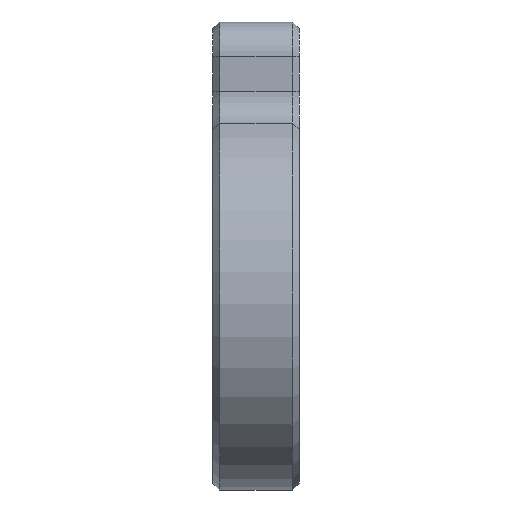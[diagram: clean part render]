
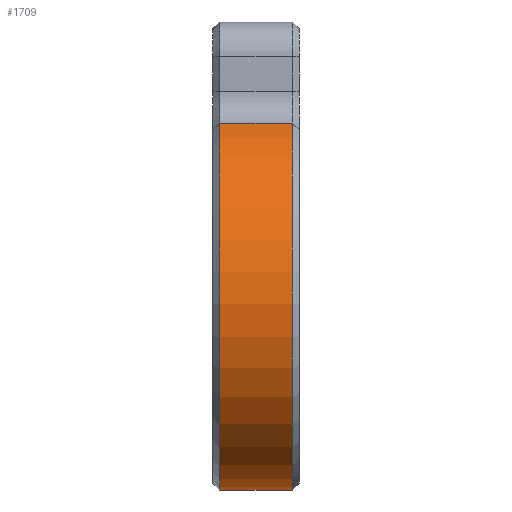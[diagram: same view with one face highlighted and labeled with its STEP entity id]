
A CAD part, front view. The second image highlights one B-rep face of the part: STEP entity #1709.
In plain terms, the highlighted cylindrical face has radius 11 mm (diameter 22 mm), a partial arc.
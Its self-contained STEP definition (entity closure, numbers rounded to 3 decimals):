
#702 = CONICAL_SURFACE('',#703,11.,0.785);
#703 = AXIS2_PLACEMENT_3D('',#704,#705,#706);
#704 = CARTESIAN_POINT('',(-2.4,0.,0.));
#705 = DIRECTION('',(-1.,-0.,0.));
#706 = DIRECTION('',(0.,0.,-1.));
#937 = CONICAL_SURFACE('',#938,11.,0.785);
#938 = AXIS2_PLACEMENT_3D('',#939,#940,#941);
#939 = CARTESIAN_POINT('',(-2.4,0.,0.));
#940 = DIRECTION('',(-1.,-0.,0.));
#941 = DIRECTION('',(0.,-0.385,0.923)
  );
#1132 = VERTEX_POINT('',#1133);
#1133 = CARTESIAN_POINT('',(-2.4,0.,-11.));
#1154 = VERTEX_POINT('',#1155);
#1155 = CARTESIAN_POINT('',(-2.4,4.231,10.154));
#1174 = EDGE_CURVE('',#1132,#1154,#1175,.T.);
#1175 = SURFACE_CURVE('',#1176,(#1181,#1188),.PCURVE_S1.);
#1176 = CIRCLE('',#1177,11.);
#1177 = AXIS2_PLACEMENT_3D('',#1178,#1179,#1180);
#1178 = CARTESIAN_POINT('',(-2.4,0.,0.));
#1179 = DIRECTION('',(1.,-0.,0.));
#1180 = DIRECTION('',(0.,0.,-1.));
#1181 = PCURVE('',#702,#1182);
#1182 = DEFINITIONAL_REPRESENTATION('',(#1183),#1187);
#1183 = LINE('',#1184,#1185);
#1184 = CARTESIAN_POINT('',(-0.,0.));
#1185 = VECTOR('',#1186,1.);
#1186 = DIRECTION('',(-1.,0.));
#1187 = ( GEOMETRIC_REPRESENTATION_CONTEXT(2) 
PARAMETRIC_REPRESENTATION_CONTEXT() REPRESENTATION_CONTEXT('2D SPACE',''
  ) );
#1188 = PCURVE('',#1189,#1194);
#1189 = CYLINDRICAL_SURFACE('',#1190,11.);
#1190 = AXIS2_PLACEMENT_3D('',#1191,#1192,#1193);
#1191 = CARTESIAN_POINT('',(-7.,0.,0.));
#1192 = DIRECTION('',(-1.,-0.,0.));
#1193 = DIRECTION('',(0.,0.,-1.));
#1194 = DEFINITIONAL_REPRESENTATION('',(#1195),#1199);
#1195 = LINE('',#1196,#1197);
#1196 = CARTESIAN_POINT('',(-6.283,-4.6));
#1197 = VECTOR('',#1198,1.);
#1198 = DIRECTION('',(-1.,0.));
#1199 = ( GEOMETRIC_REPRESENTATION_CONTEXT(2) 
PARAMETRIC_REPRESENTATION_CONTEXT() REPRESENTATION_CONTEXT('2D SPACE',''
  ) );
#1205 = VERTEX_POINT('',#1206);
#1206 = CARTESIAN_POINT('',(-2.4,-4.231,10.154));
#1227 = EDGE_CURVE('',#1205,#1132,#1228,.T.);
#1228 = SURFACE_CURVE('',#1229,(#1234,#1241),.PCURVE_S1.);
#1229 = CIRCLE('',#1230,11.);
#1230 = AXIS2_PLACEMENT_3D('',#1231,#1232,#1233);
#1231 = CARTESIAN_POINT('',(-2.4,0.,0.));
#1232 = DIRECTION('',(1.,0.,0.));
#1233 = DIRECTION('',(0.,-0.385,0.923
    ));
#1234 = PCURVE('',#937,#1235);
#1235 = DEFINITIONAL_REPRESENTATION('',(#1236),#1240);
#1236 = LINE('',#1237,#1238);
#1237 = CARTESIAN_POINT('',(-0.,0.));
#1238 = VECTOR('',#1239,1.);
#1239 = DIRECTION('',(-1.,0.));
#1240 = ( GEOMETRIC_REPRESENTATION_CONTEXT(2) 
PARAMETRIC_REPRESENTATION_CONTEXT() REPRESENTATION_CONTEXT('2D SPACE',''
  ) );
#1241 = PCURVE('',#1189,#1242);
#1242 = DEFINITIONAL_REPRESENTATION('',(#1243),#1247);
#1243 = LINE('',#1244,#1245);
#1244 = CARTESIAN_POINT('',(-3.536,-4.6));
#1245 = VECTOR('',#1246,1.);
#1246 = DIRECTION('',(-1.,0.));
#1247 = ( GEOMETRIC_REPRESENTATION_CONTEXT(2) 
PARAMETRIC_REPRESENTATION_CONTEXT() REPRESENTATION_CONTEXT('2D SPACE',''
  ) );
#1290 = CYLINDRICAL_SURFACE('',#1291,2.);
#1291 = AXIS2_PLACEMENT_3D('',#1292,#1293,#1294);
#1292 = CARTESIAN_POINT('',(-2.,5.,12.));
#1293 = DIRECTION('',(-1.,-0.,0.));
#1294 = DIRECTION('',(0.,-1.,0.));
#1343 = CYLINDRICAL_SURFACE('',#1344,2.);
#1344 = AXIS2_PLACEMENT_3D('',#1345,#1346,#1347);
#1345 = CARTESIAN_POINT('',(-2.,-5.,12.));
#1346 = DIRECTION('',(-1.,-0.,0.));
#1347 = DIRECTION('',(0.,1.,0.));
#1709 = ADVANCED_FACE('',(#1710),#1189,.T.);
#1710 = FACE_BOUND('',#1711,.F.);
#1711 = EDGE_LOOP('',(#1712,#1735,#1764,#1793,#1814,#1815));
#1712 = ORIENTED_EDGE('',*,*,#1713,.T.);
#1713 = EDGE_CURVE('',#1154,#1714,#1716,.T.);
#1714 = VERTEX_POINT('',#1715);
#1715 = CARTESIAN_POINT('',(-6.6,4.231,10.154));
#1716 = SURFACE_CURVE('',#1717,(#1721,#1728),.PCURVE_S1.);
#1717 = LINE('',#1718,#1719);
#1718 = CARTESIAN_POINT('',(-2.,4.231,10.154));
#1719 = VECTOR('',#1720,1.);
#1720 = DIRECTION('',(-1.,-0.,0.));
#1721 = PCURVE('',#1189,#1722);
#1722 = DEFINITIONAL_REPRESENTATION('',(#1723),#1727);
#1723 = LINE('',#1724,#1725);
#1724 = CARTESIAN_POINT('',(-9.03,-5.));
#1725 = VECTOR('',#1726,1.);
#1726 = DIRECTION('',(-0.,1.));
#1727 = ( GEOMETRIC_REPRESENTATION_CONTEXT(2) 
PARAMETRIC_REPRESENTATION_CONTEXT() REPRESENTATION_CONTEXT('2D SPACE',''
  ) );
#1728 = PCURVE('',#1290,#1729);
#1729 = DEFINITIONAL_REPRESENTATION('',(#1730),#1734);
#1730 = LINE('',#1731,#1732);
#1731 = CARTESIAN_POINT('',(-1.176,0.));
#1732 = VECTOR('',#1733,1.);
#1733 = DIRECTION('',(-0.,1.));
#1734 = ( GEOMETRIC_REPRESENTATION_CONTEXT(2) 
PARAMETRIC_REPRESENTATION_CONTEXT() REPRESENTATION_CONTEXT('2D SPACE',''
  ) );
#1735 = ORIENTED_EDGE('',*,*,#1736,.F.);
#1736 = EDGE_CURVE('',#1737,#1714,#1739,.T.);
#1737 = VERTEX_POINT('',#1738);
#1738 = CARTESIAN_POINT('',(-6.6,0.,-11.));
#1739 = SURFACE_CURVE('',#1740,(#1745,#1752),.PCURVE_S1.);
#1740 = CIRCLE('',#1741,11.);
#1741 = AXIS2_PLACEMENT_3D('',#1742,#1743,#1744);
#1742 = CARTESIAN_POINT('',(-6.6,0.,0.));
#1743 = DIRECTION('',(1.,-0.,0.));
#1744 = DIRECTION('',(0.,0.,-1.));
#1745 = PCURVE('',#1189,#1746);
#1746 = DEFINITIONAL_REPRESENTATION('',(#1747),#1751);
#1747 = LINE('',#1748,#1749);
#1748 = CARTESIAN_POINT('',(-6.283,-0.4));
#1749 = VECTOR('',#1750,1.);
#1750 = DIRECTION('',(-1.,0.));
#1751 = ( GEOMETRIC_REPRESENTATION_CONTEXT(2) 
PARAMETRIC_REPRESENTATION_CONTEXT() REPRESENTATION_CONTEXT('2D SPACE',''
  ) );
#1752 = PCURVE('',#1753,#1758);
#1753 = CONICAL_SURFACE('',#1754,11.,0.785);
#1754 = AXIS2_PLACEMENT_3D('',#1755,#1756,#1757);
#1755 = CARTESIAN_POINT('',(-6.6,0.,0.));
#1756 = DIRECTION('',(1.,0.,0.));
#1757 = DIRECTION('',(0.,0.,-1.));
#1758 = DEFINITIONAL_REPRESENTATION('',(#1759),#1763);
#1759 = LINE('',#1760,#1761);
#1760 = CARTESIAN_POINT('',(0.,0.));
#1761 = VECTOR('',#1762,1.);
#1762 = DIRECTION('',(1.,0.));
#1763 = ( GEOMETRIC_REPRESENTATION_CONTEXT(2) 
PARAMETRIC_REPRESENTATION_CONTEXT() REPRESENTATION_CONTEXT('2D SPACE',''
  ) );
#1764 = ORIENTED_EDGE('',*,*,#1765,.F.);
#1765 = EDGE_CURVE('',#1766,#1737,#1768,.T.);
#1766 = VERTEX_POINT('',#1767);
#1767 = CARTESIAN_POINT('',(-6.6,-4.231,10.154));
#1768 = SURFACE_CURVE('',#1769,(#1774,#1781),.PCURVE_S1.);
#1769 = CIRCLE('',#1770,11.);
#1770 = AXIS2_PLACEMENT_3D('',#1771,#1772,#1773);
#1771 = CARTESIAN_POINT('',(-6.6,0.,0.));
#1772 = DIRECTION('',(1.,0.,0.));
#1773 = DIRECTION('',(0.,-0.385,0.923
    ));
#1774 = PCURVE('',#1189,#1775);
#1775 = DEFINITIONAL_REPRESENTATION('',(#1776),#1780);
#1776 = LINE('',#1777,#1778);
#1777 = CARTESIAN_POINT('',(-3.536,-0.4));
#1778 = VECTOR('',#1779,1.);
#1779 = DIRECTION('',(-1.,0.));
#1780 = ( GEOMETRIC_REPRESENTATION_CONTEXT(2) 
PARAMETRIC_REPRESENTATION_CONTEXT() REPRESENTATION_CONTEXT('2D SPACE',''
  ) );
#1781 = PCURVE('',#1782,#1787);
#1782 = CONICAL_SURFACE('',#1783,11.,0.785);
#1783 = AXIS2_PLACEMENT_3D('',#1784,#1785,#1786);
#1784 = CARTESIAN_POINT('',(-6.6,0.,0.));
#1785 = DIRECTION('',(1.,0.,0.));
#1786 = DIRECTION('',(0.,-0.385,0.923
    ));
#1787 = DEFINITIONAL_REPRESENTATION('',(#1788),#1792);
#1788 = LINE('',#1789,#1790);
#1789 = CARTESIAN_POINT('',(0.,0.));
#1790 = VECTOR('',#1791,1.);
#1791 = DIRECTION('',(1.,0.));
#1792 = ( GEOMETRIC_REPRESENTATION_CONTEXT(2) 
PARAMETRIC_REPRESENTATION_CONTEXT() REPRESENTATION_CONTEXT('2D SPACE',''
  ) );
#1793 = ORIENTED_EDGE('',*,*,#1794,.F.);
#1794 = EDGE_CURVE('',#1205,#1766,#1795,.T.);
#1795 = SURFACE_CURVE('',#1796,(#1800,#1807),.PCURVE_S1.);
#1796 = LINE('',#1797,#1798);
#1797 = CARTESIAN_POINT('',(-2.,-4.231,10.154));
#1798 = VECTOR('',#1799,1.);
#1799 = DIRECTION('',(-1.,-0.,0.));
#1800 = PCURVE('',#1189,#1801);
#1801 = DEFINITIONAL_REPRESENTATION('',(#1802),#1806);
#1802 = LINE('',#1803,#1804);
#1803 = CARTESIAN_POINT('',(-3.536,-5.));
#1804 = VECTOR('',#1805,1.);
#1805 = DIRECTION('',(-0.,1.));
#1806 = ( GEOMETRIC_REPRESENTATION_CONTEXT(2) 
PARAMETRIC_REPRESENTATION_CONTEXT() REPRESENTATION_CONTEXT('2D SPACE',''
  ) );
#1807 = PCURVE('',#1343,#1808);
#1808 = DEFINITIONAL_REPRESENTATION('',(#1809),#1813);
#1809 = LINE('',#1810,#1811);
#1810 = CARTESIAN_POINT('',(1.176,0.));
#1811 = VECTOR('',#1812,1.);
#1812 = DIRECTION('',(0.,1.));
#1813 = ( GEOMETRIC_REPRESENTATION_CONTEXT(2) 
PARAMETRIC_REPRESENTATION_CONTEXT() REPRESENTATION_CONTEXT('2D SPACE',''
  ) );
#1814 = ORIENTED_EDGE('',*,*,#1227,.T.);
#1815 = ORIENTED_EDGE('',*,*,#1174,.T.);
